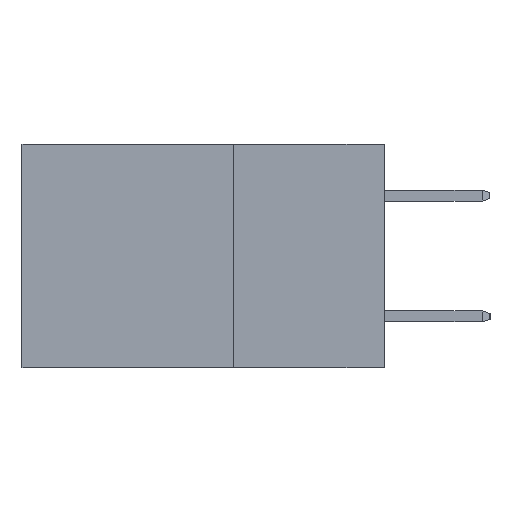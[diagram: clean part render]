
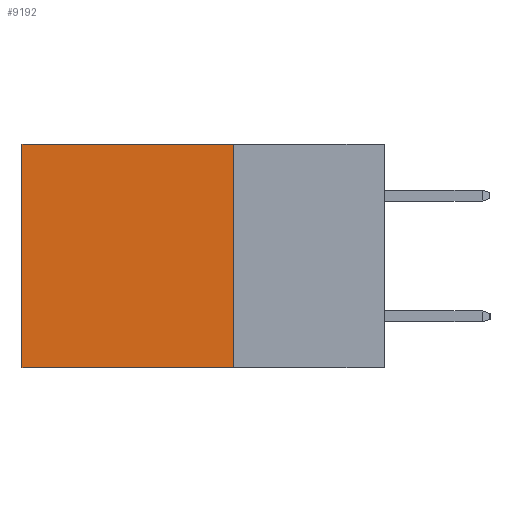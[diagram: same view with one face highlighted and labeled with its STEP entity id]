
A CAD part, left-side view. The second image highlights one B-rep face of the part: STEP entity #9192.
In plain terms, the highlighted planar face has unit normal (-1, 0, 0).
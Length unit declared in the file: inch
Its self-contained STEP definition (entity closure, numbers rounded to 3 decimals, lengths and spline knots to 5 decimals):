
#29 = VERTEX_POINT ( 'NONE', #6307 ) ;
#56 = CARTESIAN_POINT ( 'NONE',  ( 0.2615, 0.6, -0.37 ) ) ;
#305 = CARTESIAN_POINT ( 'NONE',  ( 0.2615, 0.25, -0.37 ) ) ;
#1049 = LINE ( 'NONE', #1668, #7379 ) ;
#1668 = CARTESIAN_POINT ( 'NONE',  ( 0.2615, 0.25, 0. ) ) ;
#1791 = VERTEX_POINT ( 'NONE', #14621 ) ;
#2062 = FACE_OUTER_BOUND ( 'NONE', #2079, .T. ) ;
#2079 = EDGE_LOOP ( 'NONE', ( #11519, #6139, #3196, #3243 ) ) ;
#3196 = ORIENTED_EDGE ( 'NONE', *, *, #14841, .F. ) ;
#3243 = ORIENTED_EDGE ( 'NONE', *, *, #11371, .T. ) ;
#3741 = CARTESIAN_POINT ( 'NONE',  ( 0.2615, 0.25, -0.37 ) ) ;
#3810 = CARTESIAN_POINT ( 'NONE',  ( 0.2615, 0.25, -0.37 ) ) ;
#5019 = DIRECTION ( 'NONE',  ( 1., 0., 0. ) ) ;
#6139 = ORIENTED_EDGE ( 'NONE', *, *, #10482, .F. ) ;
#6200 = LINE ( 'NONE', #3810, #16304 ) ;
#6307 = CARTESIAN_POINT ( 'NONE',  ( 0.2615, 0.25, -0.37 ) ) ;
#6734 = DIRECTION ( 'NONE',  ( 0., 1., 0. ) ) ;
#7379 = VECTOR ( 'NONE', #6734, 39.37008 ) ;
#7573 = DIRECTION ( 'NONE',  ( 0., 0., -1. ) ) ;
#8917 = DIRECTION ( 'NONE',  ( 0., 1., 0. ) ) ;
#8930 = LINE ( 'NONE', #56, #15668 ) ;
#9105 = DIRECTION ( 'NONE',  ( 0., 0., -1. ) ) ;
#9192 = ADVANCED_FACE ( 'NONE', ( #2062 ), #10009, .F. ) ;
#9935 = LINE ( 'NONE', #305, #13281 ) ;
#10009 = PLANE ( 'NONE',  #14359 ) ;
#10482 = EDGE_CURVE ( 'NONE', #29, #15854, #6200, .T. ) ;
#11371 = EDGE_CURVE ( 'NONE', #12486, #1791, #1049, .T. ) ;
#11519 = ORIENTED_EDGE ( 'NONE', *, *, #14681, .T. ) ;
#12486 = VERTEX_POINT ( 'NONE', #13530 ) ;
#12558 = CARTESIAN_POINT ( 'NONE',  ( 0.2615, 0.6, -0.37 ) ) ;
#13281 = VECTOR ( 'NONE', #9105, 39.37008 ) ;
#13530 = CARTESIAN_POINT ( 'NONE',  ( 0.2615, 0.25, 0. ) ) ;
#13865 = DIRECTION ( 'NONE',  ( 0., 0., -1. ) ) ;
#14359 = AXIS2_PLACEMENT_3D ( 'NONE', #3741, #5019, #13865 ) ;
#14621 = CARTESIAN_POINT ( 'NONE',  ( 0.2615, 0.6, 0. ) ) ;
#14681 = EDGE_CURVE ( 'NONE', #1791, #15854, #8930, .T. ) ;
#14841 = EDGE_CURVE ( 'NONE', #12486, #29, #9935, .T. ) ;
#15668 = VECTOR ( 'NONE', #7573, 39.37008 ) ;
#15854 = VERTEX_POINT ( 'NONE', #12558 ) ;
#16304 = VECTOR ( 'NONE', #8917, 39.37008 ) ;
